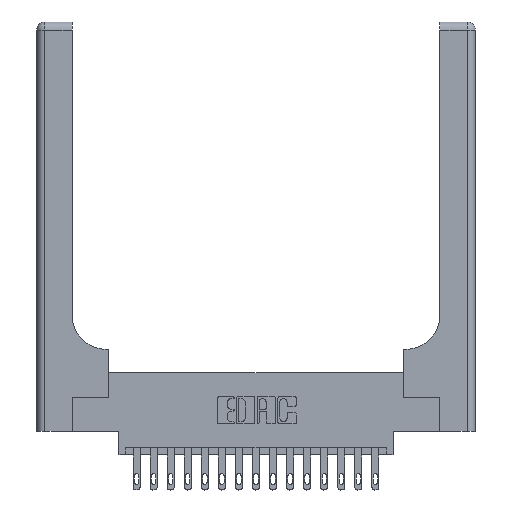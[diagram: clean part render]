
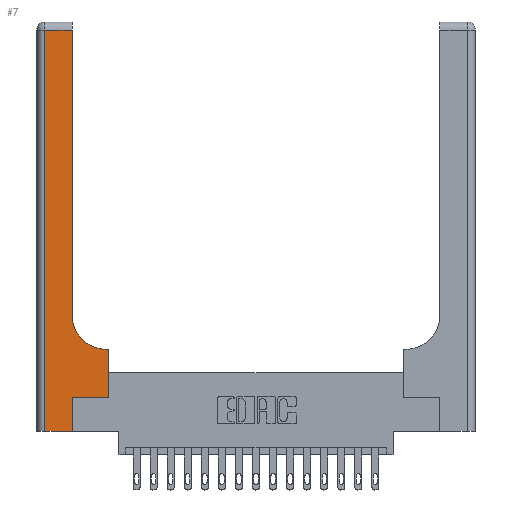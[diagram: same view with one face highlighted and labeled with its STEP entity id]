
A CAD part, top view. The second image highlights one B-rep face of the part: STEP entity #7.
In plain terms, the highlighted planar face has unit normal (0, 0, 1).
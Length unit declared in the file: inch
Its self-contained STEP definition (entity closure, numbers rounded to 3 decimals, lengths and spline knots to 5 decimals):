
#7 = ADVANCED_FACE ( 'NONE', ( #711 ), #6612, .F. ) ;
#232 = CARTESIAN_POINT ( 'NONE',  ( 0.26, 3., 0.37 ) ) ;
#302 = VERTEX_POINT ( 'NONE', #16633 ) ;
#328 = ORIENTED_EDGE ( 'NONE', *, *, #9362, .T. ) ;
#448 = VERTEX_POINT ( 'NONE', #15661 ) ;
#575 = VERTEX_POINT ( 'NONE', #18831 ) ;
#655 = VECTOR ( 'NONE', #17933, 39.37008 ) ;
#683 = VECTOR ( 'NONE', #3047, 39.37008 ) ;
#711 = FACE_OUTER_BOUND ( 'NONE', #9907, .T. ) ;
#988 = VERTEX_POINT ( 'NONE', #1311 ) ;
#1226 = EDGE_CURVE ( 'NONE', #302, #8384, #7692, .T. ) ;
#1311 = CARTESIAN_POINT ( 'NONE',  ( 0.528, 0.25, 0.37 ) ) ;
#1323 = VECTOR ( 'NONE', #12007, 39.37008 ) ;
#1499 = CARTESIAN_POINT ( 'NONE',  ( 0., 2.94, 0.37 ) ) ;
#1614 = CARTESIAN_POINT ( 'NONE',  ( 0.265, 0.25, 0.37 ) ) ;
#1637 = EDGE_CURVE ( 'NONE', #11043, #19040, #10758, .T. ) ;
#1888 = EDGE_CURVE ( 'NONE', #8384, #15937, #17807, .T. ) ;
#2691 = ORIENTED_EDGE ( 'NONE', *, *, #1637, .T. ) ;
#2979 = ORIENTED_EDGE ( 'NONE', *, *, #7724, .T. ) ;
#3047 = DIRECTION ( 'NONE',  ( -1., 0., 0. ) ) ;
#3115 = AXIS2_PLACEMENT_3D ( 'NONE', #7868, #6421, #10054 ) ;
#3310 = EDGE_CURVE ( 'NONE', #575, #9910, #4762, .T. ) ;
#3789 = VECTOR ( 'NONE', #16843, 39.37008 ) ;
#3833 = VECTOR ( 'NONE', #16264, 39.37008 ) ;
#3867 = LINE ( 'NONE', #9662, #7863 ) ;
#3966 = DIRECTION ( 'NONE',  ( 1., 0., 0. ) ) ;
#4388 = ORIENTED_EDGE ( 'NONE', *, *, #16886, .T. ) ;
#4762 = LINE ( 'NONE', #10640, #3833 ) ;
#4804 = ORIENTED_EDGE ( 'NONE', *, *, #3310, .T. ) ;
#5529 = CARTESIAN_POINT ( 'NONE',  ( 0., 3., 0.37 ) ) ;
#6421 = DIRECTION ( 'NONE',  ( 0., 0., -1. ) ) ;
#6427 = DIRECTION ( 'NONE',  ( 0., 0., -1. ) ) ;
#6515 = CIRCLE ( 'NONE', #3115, 0.25 ) ;
#6612 = PLANE ( 'NONE',  #14871 ) ;
#7329 = EDGE_CURVE ( 'NONE', #19040, #448, #6515, .T. ) ;
#7612 = VECTOR ( 'NONE', #8787, 39.37008 ) ;
#7692 = LINE ( 'NONE', #1499, #683 ) ;
#7724 = EDGE_CURVE ( 'NONE', #988, #11043, #8286, .T. ) ;
#7863 = VECTOR ( 'NONE', #3966, 39.37008 ) ;
#7868 = CARTESIAN_POINT ( 'NONE',  ( 0.51, 0.85, 0.37 ) ) ;
#7969 = ORIENTED_EDGE ( 'NONE', *, *, #14906, .T. ) ;
#8273 = CARTESIAN_POINT ( 'NONE',  ( 0.528, 0.6, 0.37 ) ) ;
#8286 = LINE ( 'NONE', #11572, #8326 ) ;
#8326 = VECTOR ( 'NONE', #17276, 39.37008 ) ;
#8384 = VERTEX_POINT ( 'NONE', #12765 ) ;
#8590 = ORIENTED_EDGE ( 'NONE', *, *, #1888, .T. ) ;
#8787 = DIRECTION ( 'NONE',  ( 1., 0., 0. ) ) ;
#9362 = EDGE_CURVE ( 'NONE', #448, #302, #12034, .T. ) ;
#9662 = CARTESIAN_POINT ( 'NONE',  ( 0., 0., 0.37 ) ) ;
#9907 = EDGE_LOOP ( 'NONE', ( #328, #12608, #8590, #7969, #4804, #4388, #2979, #2691, #17038 ) ) ;
#9910 = VERTEX_POINT ( 'NONE', #18752 ) ;
#9978 = DIRECTION ( 'NONE',  ( -1., 0., 0. ) ) ;
#10054 = DIRECTION ( 'NONE',  ( 1., 0., 0. ) ) ;
#10640 = CARTESIAN_POINT ( 'NONE',  ( 0.265, 0., 0.37 ) ) ;
#10758 = LINE ( 'NONE', #13757, #3789 ) ;
#11043 = VERTEX_POINT ( 'NONE', #8273 ) ;
#11572 = CARTESIAN_POINT ( 'NONE',  ( 0.528, 0.25, 0.37 ) ) ;
#11842 = CARTESIAN_POINT ( 'NONE',  ( 0.51, 0.6, 0.37 ) ) ;
#12007 = DIRECTION ( 'NONE',  ( 0., -1., 0. ) ) ;
#12034 = LINE ( 'NONE', #232, #655 ) ;
#12608 = ORIENTED_EDGE ( 'NONE', *, *, #1226, .T. ) ;
#12765 = CARTESIAN_POINT ( 'NONE',  ( 0.06, 2.94, 0.37 ) ) ;
#13757 = CARTESIAN_POINT ( 'NONE',  ( 0.26, 0.6, 0.37 ) ) ;
#14871 = AXIS2_PLACEMENT_3D ( 'NONE', #5529, #6427, #9978 ) ;
#14906 = EDGE_CURVE ( 'NONE', #15937, #575, #3867, .T. ) ;
#15635 = CARTESIAN_POINT ( 'NONE',  ( 0.06, 0., 0.37 ) ) ;
#15661 = CARTESIAN_POINT ( 'NONE',  ( 0.26, 0.85, 0.37 ) ) ;
#15937 = VERTEX_POINT ( 'NONE', #15635 ) ;
#16264 = DIRECTION ( 'NONE',  ( 0., 1., 0. ) ) ;
#16522 = LINE ( 'NONE', #1614, #7612 ) ;
#16633 = CARTESIAN_POINT ( 'NONE',  ( 0.26, 2.94, 0.37 ) ) ;
#16801 = CARTESIAN_POINT ( 'NONE',  ( 0.06, 3., 0.37 ) ) ;
#16843 = DIRECTION ( 'NONE',  ( -1., 0., 0. ) ) ;
#16886 = EDGE_CURVE ( 'NONE', #9910, #988, #16522, .T. ) ;
#17038 = ORIENTED_EDGE ( 'NONE', *, *, #7329, .T. ) ;
#17276 = DIRECTION ( 'NONE',  ( 0., 1., 0. ) ) ;
#17807 = LINE ( 'NONE', #16801, #1323 ) ;
#17933 = DIRECTION ( 'NONE',  ( 0., 1., 0. ) ) ;
#18752 = CARTESIAN_POINT ( 'NONE',  ( 0.265, 0.25, 0.37 ) ) ;
#18831 = CARTESIAN_POINT ( 'NONE',  ( 0.265, 0., 0.37 ) ) ;
#19040 = VERTEX_POINT ( 'NONE', #11842 ) ;
